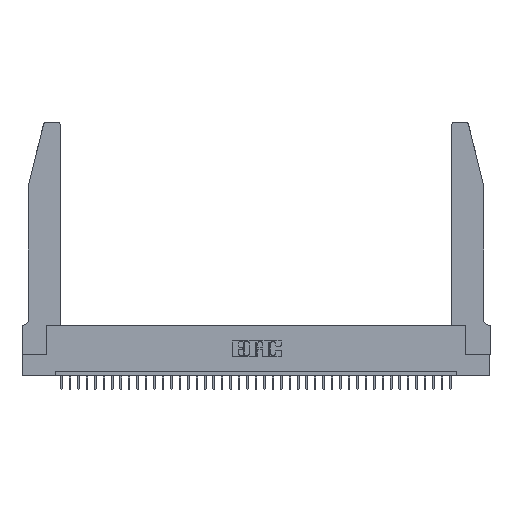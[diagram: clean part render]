
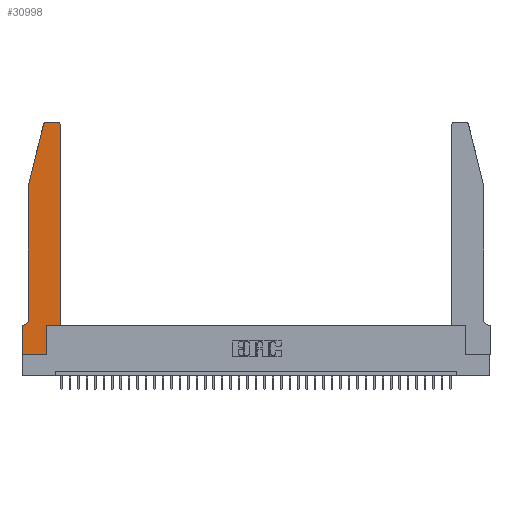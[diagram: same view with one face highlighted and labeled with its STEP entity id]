
A CAD part, top view. The second image highlights one B-rep face of the part: STEP entity #30998.
In plain terms, the highlighted planar face has unit normal (0, 0, 1).
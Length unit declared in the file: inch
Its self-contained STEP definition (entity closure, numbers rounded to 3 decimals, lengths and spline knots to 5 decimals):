
#354 = EDGE_CURVE ( 'NONE', #1284, #25488, #8425, .T. ) ;
#372 = CARTESIAN_POINT ( 'NONE',  ( 0.25487, 2.72718, 0.37 ) ) ;
#636 = CARTESIAN_POINT ( 'NONE',  ( 0.0055, 0.42, 0.37 ) ) ;
#1284 = VERTEX_POINT ( 'NONE', #37715 ) ;
#1505 = VERTEX_POINT ( 'NONE', #34608 ) ;
#1518 = VERTEX_POINT ( 'NONE', #7833 ) ;
#1664 = ORIENTED_EDGE ( 'NONE', *, *, #4070, .T. ) ;
#1876 = LINE ( 'NONE', #26782, #36697 ) ;
#1908 = CIRCLE ( 'NONE', #5937, 0.07 ) ;
#1933 = EDGE_CURVE ( 'NONE', #28863, #38854, #3636, .T. ) ;
#2070 = AXIS2_PLACEMENT_3D ( 'NONE', #24032, #33148, #32619 ) ;
#2233 = DIRECTION ( 'NONE',  ( 1., 0., 0. ) ) ;
#2234 = CARTESIAN_POINT ( 'NONE',  ( 0., 0.35, 0.37 ) ) ;
#3224 = LINE ( 'NONE', #32105, #3658 ) ;
#3636 = LINE ( 'NONE', #26825, #35215 ) ;
#3658 = VECTOR ( 'NONE', #4331, 39.37008 ) ;
#3724 = DIRECTION ( 'NONE',  ( 0., 0., -1. ) ) ;
#4070 = EDGE_CURVE ( 'NONE', #19700, #1505, #26408, .T. ) ;
#4331 = DIRECTION ( 'NONE',  ( 0., -1., 0. ) ) ;
#4761 = CARTESIAN_POINT ( 'NONE',  ( 0.0755, 2., 0.37 ) ) ;
#4881 = ORIENTED_EDGE ( 'NONE', *, *, #354, .T. ) ;
#5129 = ORIENTED_EDGE ( 'NONE', *, *, #37142, .T. ) ;
#5425 = DIRECTION ( 'NONE',  ( 0., -1., 0. ) ) ;
#5937 = AXIS2_PLACEMENT_3D ( 'NONE', #636, #3724, #30546 ) ;
#6855 = DIRECTION ( 'NONE',  ( 1., 0., 0. ) ) ;
#7185 = FACE_OUTER_BOUND ( 'NONE', #27522, .T. ) ;
#7341 = CARTESIAN_POINT ( 'NONE',  ( 0.4505, 0.35, 0.37 ) ) ;
#7471 = ORIENTED_EDGE ( 'NONE', *, *, #13534, .T. ) ;
#7833 = CARTESIAN_POINT ( 'NONE',  ( 0.0755, 2., 0.37 ) ) ;
#8425 = CIRCLE ( 'NONE', #26153, 0.03 ) ;
#10953 = VECTOR ( 'NONE', #5425, 39.37008 ) ;
#11771 = CARTESIAN_POINT ( 'NONE',  ( 0.4505, 2.72, 0.37 ) ) ;
#12049 = EDGE_CURVE ( 'NONE', #25488, #1518, #35770, .T. ) ;
#13230 = DIRECTION ( 'NONE',  ( 0., 0., 1. ) ) ;
#13534 = EDGE_CURVE ( 'NONE', #22677, #19700, #19157, .T. ) ;
#14232 = VECTOR ( 'NONE', #21013, 39.37008 ) ;
#15081 = VERTEX_POINT ( 'NONE', #30789 ) ;
#15270 = ORIENTED_EDGE ( 'NONE', *, *, #24699, .T. ) ;
#15548 = CARTESIAN_POINT ( 'NONE',  ( 0.4505, 0.35, 0.37 ) ) ;
#15577 = LINE ( 'NONE', #36789, #22753 ) ;
#16228 = AXIS2_PLACEMENT_3D ( 'NONE', #28196, #13230, #6855 ) ;
#17766 = ORIENTED_EDGE ( 'NONE', *, *, #25053, .T. ) ;
#18313 = DIRECTION ( 'NONE',  ( -1., 0., 0. ) ) ;
#18912 = VECTOR ( 'NONE', #27121, 39.37008 ) ;
#19157 = LINE ( 'NONE', #15548, #26385 ) ;
#19700 = VERTEX_POINT ( 'NONE', #11771 ) ;
#21013 = DIRECTION ( 'NONE',  ( 1., 0., 0. ) ) ;
#21422 = ORIENTED_EDGE ( 'NONE', *, *, #23692, .T. ) ;
#21649 = ORIENTED_EDGE ( 'NONE', *, *, #31853, .T. ) ;
#22117 = CARTESIAN_POINT ( 'NONE',  ( 0.0055, 0.35, 0.37 ) ) ;
#22279 = LINE ( 'NONE', #27653, #14232 ) ;
#22677 = VERTEX_POINT ( 'NONE', #7341 ) ;
#22753 = VECTOR ( 'NONE', #18313, 39.37008 ) ;
#22842 = ORIENTED_EDGE ( 'NONE', *, *, #1933, .T. ) ;
#23692 = EDGE_CURVE ( 'NONE', #37905, #28863, #1908, .T. ) ;
#23721 = CARTESIAN_POINT ( 'NONE',  ( 0.284, 2.72, 0.37 ) ) ;
#23917 = CARTESIAN_POINT ( 'NONE',  ( 0.2865, 0.35, 0.37 ) ) ;
#24032 = CARTESIAN_POINT ( 'NONE',  ( 0., 0.35, 0.37 ) ) ;
#24289 = EDGE_CURVE ( 'NONE', #15081, #24715, #24725, .T. ) ;
#24568 = EDGE_CURVE ( 'NONE', #24715, #27088, #1876, .T. ) ;
#24699 = EDGE_CURVE ( 'NONE', #27088, #22677, #22279, .T. ) ;
#24715 = VERTEX_POINT ( 'NONE', #27396 ) ;
#24725 = LINE ( 'NONE', #38005, #30018 ) ;
#24920 = ORIENTED_EDGE ( 'NONE', *, *, #12049, .T. ) ;
#25053 = EDGE_CURVE ( 'NONE', #38854, #15081, #3224, .T. ) ;
#25260 = ORIENTED_EDGE ( 'NONE', *, *, #24568, .T. ) ;
#25488 = VERTEX_POINT ( 'NONE', #372 ) ;
#26153 = AXIS2_PLACEMENT_3D ( 'NONE', #23721, #36018, #2233 ) ;
#26385 = VECTOR ( 'NONE', #34416, 39.37008 ) ;
#26408 = CIRCLE ( 'NONE', #16228, 0.03 ) ;
#26782 = CARTESIAN_POINT ( 'NONE',  ( 0.2865, 0.35, 0.37 ) ) ;
#26825 = CARTESIAN_POINT ( 'NONE',  ( 0.0755, 0.35, 0.37 ) ) ;
#27088 = VERTEX_POINT ( 'NONE', #23917 ) ;
#27121 = DIRECTION ( 'NONE',  ( -0.239, -0.971, 0. ) ) ;
#27210 = LINE ( 'NONE', #32774, #10953 ) ;
#27396 = CARTESIAN_POINT ( 'NONE',  ( 0.2865, 0., 0.37 ) ) ;
#27522 = EDGE_LOOP ( 'NONE', ( #5129, #4881, #24920, #21649, #21422, #22842, #17766, #38420, #25260, #15270, #7471, #1664 ) ) ;
#27653 = CARTESIAN_POINT ( 'NONE',  ( 0.4505, 0.35, 0.37 ) ) ;
#27925 = DIRECTION ( 'NONE',  ( 1., 0., 0. ) ) ;
#28196 = CARTESIAN_POINT ( 'NONE',  ( 0.4205, 2.72, 0.37 ) ) ;
#28863 = VERTEX_POINT ( 'NONE', #22117 ) ;
#29707 = DIRECTION ( 'NONE',  ( 0., 1., 0. ) ) ;
#29891 = DIRECTION ( 'NONE',  ( -1., 0., 0. ) ) ;
#30018 = VECTOR ( 'NONE', #27925, 39.37008 ) ;
#30546 = DIRECTION ( 'NONE',  ( -1., 0., 0. ) ) ;
#30789 = CARTESIAN_POINT ( 'NONE',  ( 0., 0., 0.37 ) ) ;
#30998 = ADVANCED_FACE ( 'NONE', ( #7185 ), #32743, .T. ) ;
#31853 = EDGE_CURVE ( 'NONE', #1518, #37905, #27210, .T. ) ;
#32105 = CARTESIAN_POINT ( 'NONE',  ( 0., 0., 0.37 ) ) ;
#32619 = DIRECTION ( 'NONE',  ( 1., 0., 0. ) ) ;
#32743 = PLANE ( 'NONE',  #2070 ) ;
#32774 = CARTESIAN_POINT ( 'NONE',  ( 0.0755, 2., 0.37 ) ) ;
#33148 = DIRECTION ( 'NONE',  ( 0., 0., 1. ) ) ;
#34281 = CARTESIAN_POINT ( 'NONE',  ( 0.0755, 0.42, 0.37 ) ) ;
#34416 = DIRECTION ( 'NONE',  ( 0., 1., 0. ) ) ;
#34608 = CARTESIAN_POINT ( 'NONE',  ( 0.4205, 2.75, 0.37 ) ) ;
#35215 = VECTOR ( 'NONE', #29891, 39.37008 ) ;
#35770 = LINE ( 'NONE', #4761, #18912 ) ;
#36018 = DIRECTION ( 'NONE',  ( 0., 0., 1. ) ) ;
#36697 = VECTOR ( 'NONE', #29707, 39.37008 ) ;
#36789 = CARTESIAN_POINT ( 'NONE',  ( 0.2605, 2.75, 0.37 ) ) ;
#37142 = EDGE_CURVE ( 'NONE', #1505, #1284, #15577, .T. ) ;
#37715 = CARTESIAN_POINT ( 'NONE',  ( 0.284, 2.75, 0.37 ) ) ;
#37905 = VERTEX_POINT ( 'NONE', #34281 ) ;
#38005 = CARTESIAN_POINT ( 'NONE',  ( 0., 0., 0.37 ) ) ;
#38420 = ORIENTED_EDGE ( 'NONE', *, *, #24289, .T. ) ;
#38854 = VERTEX_POINT ( 'NONE', #2234 ) ;
